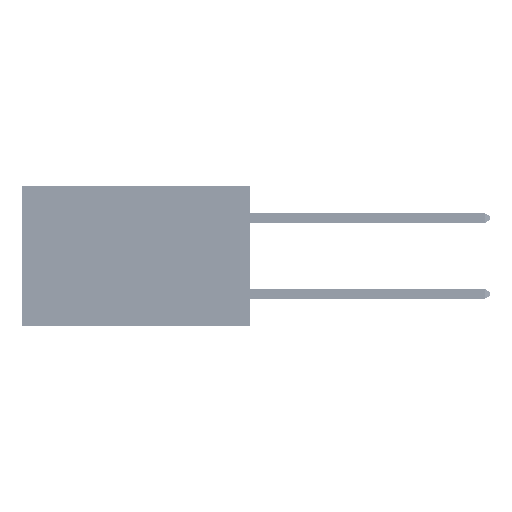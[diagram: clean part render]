
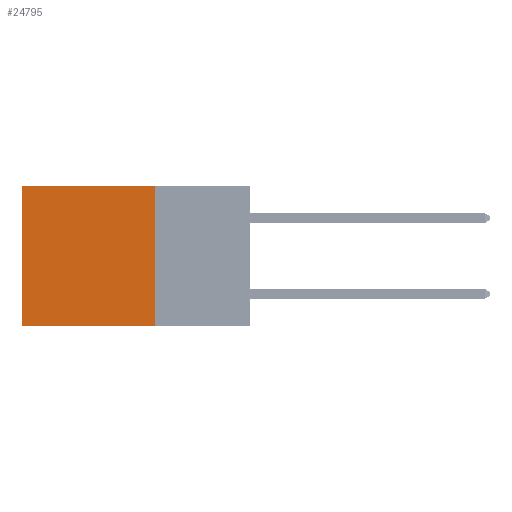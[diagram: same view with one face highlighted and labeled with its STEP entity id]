
A CAD part, left-side view. The second image highlights one B-rep face of the part: STEP entity #24795.
In plain terms, the highlighted planar face has unit normal (-1, 0, 0).
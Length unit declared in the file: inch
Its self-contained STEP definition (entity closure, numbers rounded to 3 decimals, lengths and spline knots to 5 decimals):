
#1818 = VERTEX_POINT ( 'NONE', #2092 ) ;
#2092 = CARTESIAN_POINT ( 'NONE',  ( 0.2875, 0.25, -0.37 ) ) ;
#4242 = CARTESIAN_POINT ( 'NONE',  ( 0.2875, 0.25, 0. ) ) ;
#4368 = EDGE_CURVE ( 'NONE', #12982, #1818, #44089, .T. ) ;
#7571 = CARTESIAN_POINT ( 'NONE',  ( 0.2875, 0.25, -0.37 ) ) ;
#7690 = CARTESIAN_POINT ( 'NONE',  ( 0.2875, 0.25, 0. ) ) ;
#7880 = EDGE_LOOP ( 'NONE', ( #27331, #41808, #14556, #45094 ) ) ;
#9134 = LINE ( 'NONE', #7571, #31986 ) ;
#12428 = FACE_OUTER_BOUND ( 'NONE', #7880, .T. ) ;
#12982 = VERTEX_POINT ( 'NONE', #46117 ) ;
#14340 = DIRECTION ( 'NONE',  ( 0., 0., -1. ) ) ;
#14556 = ORIENTED_EDGE ( 'NONE', *, *, #4368, .F. ) ;
#15292 = CARTESIAN_POINT ( 'NONE',  ( 0.2875, 0.6, -0.37 ) ) ;
#17027 = VERTEX_POINT ( 'NONE', #41768 ) ;
#23639 = EDGE_CURVE ( 'NONE', #12982, #17027, #24275, .T. ) ;
#24275 = LINE ( 'NONE', #7690, #24884 ) ;
#24795 = ADVANCED_FACE ( 'NONE', ( #12428 ), #40343, .F. ) ;
#24884 = VECTOR ( 'NONE', #45481, 39.37008 ) ;
#27171 = VECTOR ( 'NONE', #40870, 39.37008 ) ;
#27331 = ORIENTED_EDGE ( 'NONE', *, *, #29628, .T. ) ;
#28274 = VECTOR ( 'NONE', #37498, 39.37008 ) ;
#29217 = DIRECTION ( 'NONE',  ( 1., 0., 0. ) ) ;
#29628 = EDGE_CURVE ( 'NONE', #17027, #40344, #47091, .T. ) ;
#30869 = AXIS2_PLACEMENT_3D ( 'NONE', #43954, #29217, #14340 ) ;
#31986 = VECTOR ( 'NONE', #36035, 39.37008 ) ;
#34181 = EDGE_CURVE ( 'NONE', #1818, #40344, #9134, .T. ) ;
#36035 = DIRECTION ( 'NONE',  ( 0., 1., 0. ) ) ;
#37498 = DIRECTION ( 'NONE',  ( 0., 0., -1. ) ) ;
#40343 = PLANE ( 'NONE',  #30869 ) ;
#40344 = VERTEX_POINT ( 'NONE', #15292 ) ;
#40870 = DIRECTION ( 'NONE',  ( 0., 0., -1. ) ) ;
#41768 = CARTESIAN_POINT ( 'NONE',  ( 0.2875, 0.6, 0. ) ) ;
#41808 = ORIENTED_EDGE ( 'NONE', *, *, #34181, .F. ) ;
#43954 = CARTESIAN_POINT ( 'NONE',  ( 0.2875, 0.25, 0. ) ) ;
#44089 = LINE ( 'NONE', #4242, #28274 ) ;
#44624 = CARTESIAN_POINT ( 'NONE',  ( 0.2875, 0.6, 0. ) ) ;
#45094 = ORIENTED_EDGE ( 'NONE', *, *, #23639, .T. ) ;
#45481 = DIRECTION ( 'NONE',  ( 0., 1., 0. ) ) ;
#46117 = CARTESIAN_POINT ( 'NONE',  ( 0.2875, 0.25, 0. ) ) ;
#47091 = LINE ( 'NONE', #44624, #27171 ) ;
